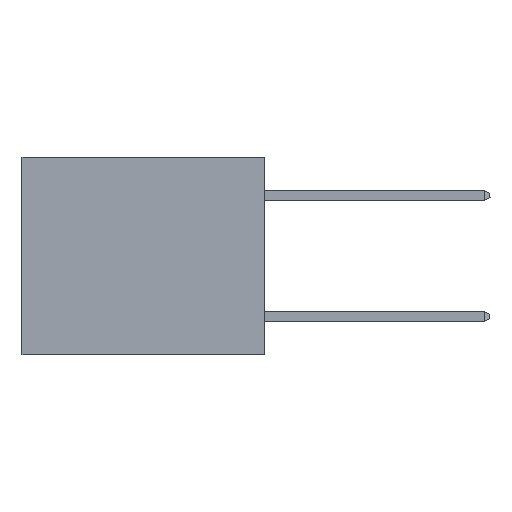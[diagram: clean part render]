
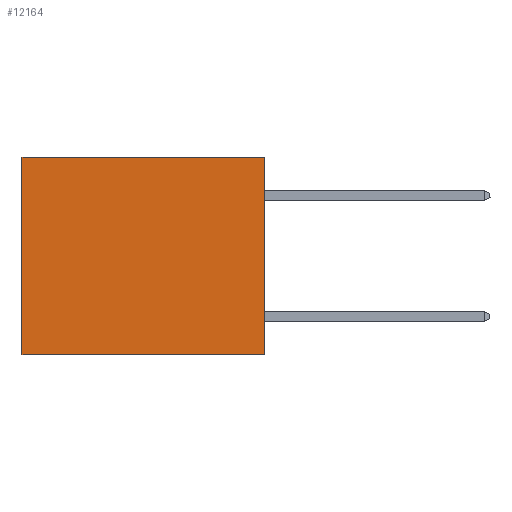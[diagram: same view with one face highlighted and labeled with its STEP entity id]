
A CAD part, left-side view. The second image highlights one B-rep face of the part: STEP entity #12164.
In plain terms, the highlighted planar face has unit normal (-1, 0, 0).
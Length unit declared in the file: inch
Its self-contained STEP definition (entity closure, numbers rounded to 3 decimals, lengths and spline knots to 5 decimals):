
#1354 = CARTESIAN_POINT ( 'NONE',  ( 0.3165, 0., -0.49 ) ) ;
#1919 = EDGE_CURVE ( 'NONE', #8513, #10178, #14138, .T. ) ;
#3625 = ORIENTED_EDGE ( 'NONE', *, *, #1919, .T. ) ;
#3647 = CARTESIAN_POINT ( 'NONE',  ( 0.3165, 0., 0. ) ) ;
#3831 = CARTESIAN_POINT ( 'NONE',  ( 0.3165, 0., -0.49 ) ) ;
#4133 = DIRECTION ( 'NONE',  ( 0., 0., -1. ) ) ;
#4250 = ORIENTED_EDGE ( 'NONE', *, *, #22338, .F. ) ;
#5186 = DIRECTION ( 'NONE',  ( 0., 1., 0. ) ) ;
#6260 = CARTESIAN_POINT ( 'NONE',  ( 0.3165, 0.6, -0.49 ) ) ;
#6287 = AXIS2_PLACEMENT_3D ( 'NONE', #1354, #18965, #8407 ) ;
#6588 = ORIENTED_EDGE ( 'NONE', *, *, #9800, .F. ) ;
#7874 = LINE ( 'NONE', #8184, #8415 ) ;
#8184 = CARTESIAN_POINT ( 'NONE',  ( 0.3165, 0.6, -0.49 ) ) ;
#8407 = DIRECTION ( 'NONE',  ( 0., 0., -1. ) ) ;
#8415 = VECTOR ( 'NONE', #20640, 39.37008 ) ;
#8513 = VERTEX_POINT ( 'NONE', #19553 ) ;
#8779 = LINE ( 'NONE', #20504, #17555 ) ;
#8885 = VECTOR ( 'NONE', #4133, 39.37008 ) ;
#9371 = CARTESIAN_POINT ( 'NONE',  ( 0.3165, 0., -0.49 ) ) ;
#9800 = EDGE_CURVE ( 'NONE', #14064, #15897, #8779, .T. ) ;
#9880 = DIRECTION ( 'NONE',  ( 0., 1., 0. ) ) ;
#10178 = VERTEX_POINT ( 'NONE', #12005 ) ;
#10789 = LINE ( 'NONE', #9371, #8885 ) ;
#11426 = VECTOR ( 'NONE', #5186, 39.37008 ) ;
#11541 = EDGE_CURVE ( 'NONE', #10178, #15897, #7874, .T. ) ;
#12005 = CARTESIAN_POINT ( 'NONE',  ( 0.3165, 0.6, 0. ) ) ;
#12164 = ADVANCED_FACE ( 'NONE', ( #15512 ), #17308, .F. ) ;
#14064 = VERTEX_POINT ( 'NONE', #3831 ) ;
#14138 = LINE ( 'NONE', #3647, #11426 ) ;
#15512 = FACE_OUTER_BOUND ( 'NONE', #17678, .T. ) ;
#15897 = VERTEX_POINT ( 'NONE', #6260 ) ;
#17308 = PLANE ( 'NONE',  #6287 ) ;
#17555 = VECTOR ( 'NONE', #9880, 39.37008 ) ;
#17678 = EDGE_LOOP ( 'NONE', ( #22468, #6588, #4250, #3625 ) ) ;
#18965 = DIRECTION ( 'NONE',  ( 1., 0., 0. ) ) ;
#19553 = CARTESIAN_POINT ( 'NONE',  ( 0.3165, 0., 0. ) ) ;
#20504 = CARTESIAN_POINT ( 'NONE',  ( 0.3165, 0., -0.49 ) ) ;
#20640 = DIRECTION ( 'NONE',  ( 0., 0., -1. ) ) ;
#22338 = EDGE_CURVE ( 'NONE', #8513, #14064, #10789, .T. ) ;
#22468 = ORIENTED_EDGE ( 'NONE', *, *, #11541, .T. ) ;
